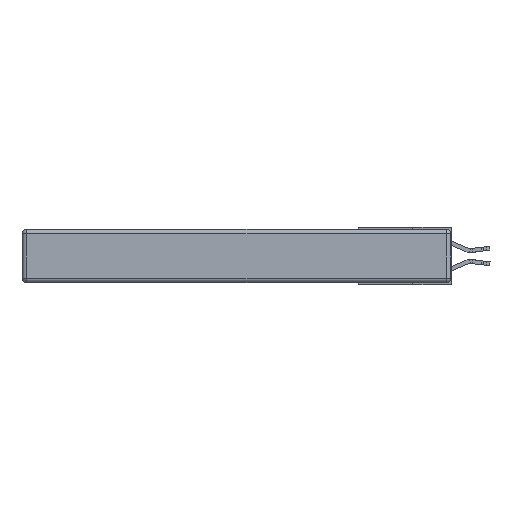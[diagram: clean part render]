
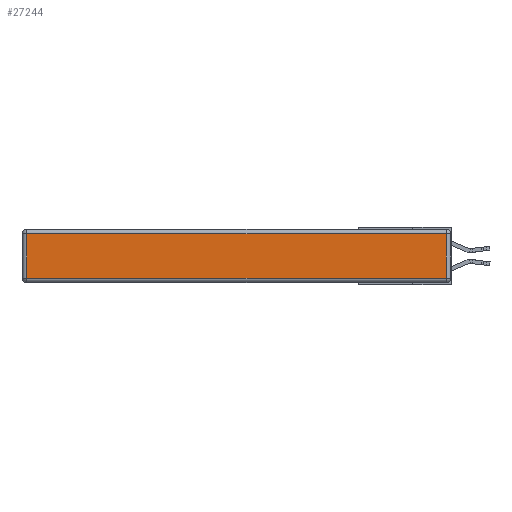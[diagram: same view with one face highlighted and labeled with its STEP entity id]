
A CAD part, left-side view. The second image highlights one B-rep face of the part: STEP entity #27244.
In plain terms, the highlighted planar face has unit normal (-1, 0, 0).
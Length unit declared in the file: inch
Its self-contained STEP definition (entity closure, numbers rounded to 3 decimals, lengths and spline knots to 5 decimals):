
#1506 = VERTEX_POINT ( 'NONE', #24207 ) ;
#4603 = VECTOR ( 'NONE', #19666, 39.37008 ) ;
#5391 = VECTOR ( 'NONE', #24879, 39.37008 ) ;
#6279 = CARTESIAN_POINT ( 'NONE',  ( 0., 0.03, -0.03 ) ) ;
#6895 = EDGE_CURVE ( 'NONE', #25396, #1506, #18477, .T. ) ;
#7262 = DIRECTION ( 'NONE',  ( 0., 0., -1. ) ) ;
#8488 = ORIENTED_EDGE ( 'NONE', *, *, #6895, .T. ) ;
#8690 = VERTEX_POINT ( 'NONE', #30179 ) ;
#10052 = EDGE_CURVE ( 'NONE', #1506, #8690, #29295, .T. ) ;
#10620 = CARTESIAN_POINT ( 'NONE',  ( 0., 0., -0.343 ) ) ;
#11897 = CARTESIAN_POINT ( 'NONE',  ( 0., 2.75, -0.03 ) ) ;
#12611 = ORIENTED_EDGE ( 'NONE', *, *, #22889, .T. ) ;
#14582 = VECTOR ( 'NONE', #16167, 39.37008 ) ;
#14932 = CARTESIAN_POINT ( 'NONE',  ( 0., 2.72, -0.343 ) ) ;
#16167 = DIRECTION ( 'NONE',  ( 0., -1., 0. ) ) ;
#17722 = VERTEX_POINT ( 'NONE', #21891 ) ;
#18228 = LINE ( 'NONE', #24264, #14582 ) ;
#18477 = LINE ( 'NONE', #11897, #4603 ) ;
#19666 = DIRECTION ( 'NONE',  ( 0., 1., 0. ) ) ;
#20140 = FACE_OUTER_BOUND ( 'NONE', #27249, .T. ) ;
#20907 = LINE ( 'NONE', #27277, #5391 ) ;
#21891 = CARTESIAN_POINT ( 'NONE',  ( 0., 0.03, -0.313 ) ) ;
#22368 = VECTOR ( 'NONE', #7262, 39.37008 ) ;
#22889 = EDGE_CURVE ( 'NONE', #8690, #17722, #18228, .T. ) ;
#24207 = CARTESIAN_POINT ( 'NONE',  ( 0., 2.72, -0.03 ) ) ;
#24219 = ORIENTED_EDGE ( 'NONE', *, *, #31166, .T. ) ;
#24264 = CARTESIAN_POINT ( 'NONE',  ( 0., 0., -0.313 ) ) ;
#24498 = ORIENTED_EDGE ( 'NONE', *, *, #10052, .T. ) ;
#24879 = DIRECTION ( 'NONE',  ( 0., 0., 1. ) ) ;
#25396 = VERTEX_POINT ( 'NONE', #6279 ) ;
#26381 = DIRECTION ( 'NONE',  ( -1., 0., 0. ) ) ;
#27244 = ADVANCED_FACE ( 'NONE', ( #20140 ), #29117, .T. ) ;
#27249 = EDGE_LOOP ( 'NONE', ( #12611, #24219, #8488, #24498 ) ) ;
#27277 = CARTESIAN_POINT ( 'NONE',  ( 0., 0.03, -0.343 ) ) ;
#29117 = PLANE ( 'NONE',  #32614 ) ;
#29295 = LINE ( 'NONE', #14932, #22368 ) ;
#30179 = CARTESIAN_POINT ( 'NONE',  ( 0., 2.72, -0.313 ) ) ;
#31166 = EDGE_CURVE ( 'NONE', #17722, #25396, #20907, .T. ) ;
#31727 = DIRECTION ( 'NONE',  ( 0., 0., 1. ) ) ;
#32614 = AXIS2_PLACEMENT_3D ( 'NONE', #10620, #26381, #31727 ) ;
